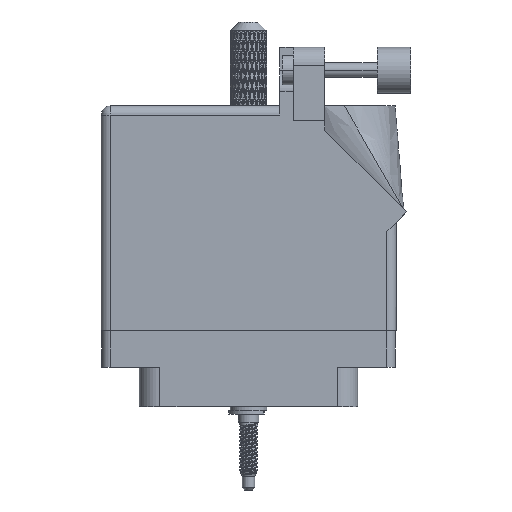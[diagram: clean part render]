
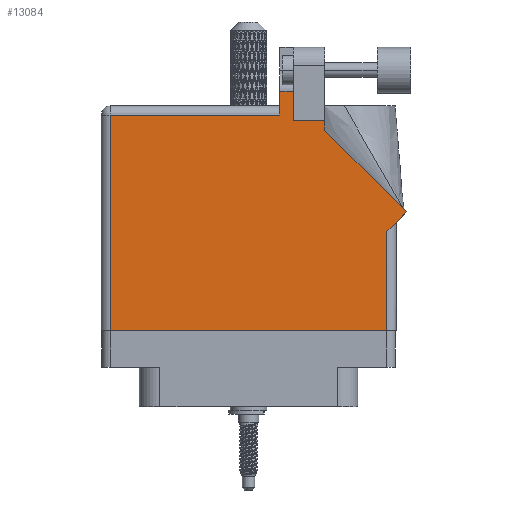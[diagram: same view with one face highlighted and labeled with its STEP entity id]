
A CAD part, front view. The second image highlights one B-rep face of the part: STEP entity #13084.
In plain terms, the highlighted face is planar.
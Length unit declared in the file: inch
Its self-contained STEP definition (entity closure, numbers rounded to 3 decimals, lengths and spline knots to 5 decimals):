
#128 = VERTEX_POINT ( 'NONE', #26891 ) ;
#2565 = EDGE_CURVE ( 'NONE', #128, #59512, #86111, .T. ) ;
#3086 = DIRECTION ( 'NONE',  ( 0.707, 0.707, 0. ) ) ;
#4726 = CARTESIAN_POINT ( 'NONE',  ( 0.519, 1.26442, 0.455 ) ) ;
#7536 = DIRECTION ( 'NONE',  ( 0., 0., -1. ) ) ;
#7722 = ORIENTED_EDGE ( 'NONE', *, *, #2565, .T. ) ;
#7923 = LINE ( 'NONE', #4726, #43890 ) ;
#8222 = LINE ( 'NONE', #74037, #45433 ) ;
#8623 = VECTOR ( 'NONE', #84389, 39.37008 ) ;
#8943 = EDGE_CURVE ( 'NONE', #104145, #89883, #28456, .T. ) ;
#11627 = EDGE_LOOP ( 'NONE', ( #90896, #99315, #51943, #72478, #7722, #75152, #79350, #53015, #60613, #103608, #106268 ) ) ;
#13084 = ADVANCED_FACE ( 'NONE', ( #33211 ), #72711, .F. ) ;
#14234 = CARTESIAN_POINT ( 'NONE',  ( 0.519, 1.33, 0.455 ) ) ;
#14616 = EDGE_CURVE ( 'NONE', #39354, #104145, #7923, .T. ) ;
#15587 = VECTOR ( 'NONE', #35825, 39.37008 ) ;
#15795 = DIRECTION ( 'NONE',  ( -1., 0., 0. ) ) ;
#16015 = EDGE_CURVE ( 'NONE', #94150, #39354, #99330, .T. ) ;
#16647 = EDGE_CURVE ( 'NONE', #42135, #82045, #8222, .T. ) ;
#16929 = CARTESIAN_POINT ( 'NONE',  ( 0.212, 1.368, 0.455 ) ) ;
#19706 = CARTESIAN_POINT ( 'NONE',  ( -0.943, -0.1, 0.455 ) ) ;
#22257 = VERTEX_POINT ( 'NONE', #84050 ) ;
#22921 = CARTESIAN_POINT ( 'NONE',  ( -1.005, 1.43, 0.455 ) ) ;
#24423 = EDGE_CURVE ( 'NONE', #89883, #22257, #54554, .T. ) ;
#24995 = DIRECTION ( 'NONE',  ( 0., 1., 0. ) ) ;
#25108 = EDGE_CURVE ( 'NONE', #73264, #42412, #90518, .T. ) ;
#26891 = CARTESIAN_POINT ( 'NONE',  ( -0.943, 1.368, 0.455 ) ) ;
#28456 = LINE ( 'NONE', #14234, #105423 ) ;
#32043 = CARTESIAN_POINT ( 'NONE',  ( 0.212, 1.43, 0.455 ) ) ;
#33211 = FACE_OUTER_BOUND ( 'NONE', #11627, .T. ) ;
#33916 = VECTOR ( 'NONE', #79499, 39.37008 ) ;
#35825 = DIRECTION ( 'NONE',  ( 0., -1., 0. ) ) ;
#36109 = EDGE_CURVE ( 'NONE', #82045, #94150, #38655, .T. ) ;
#37940 = VECTOR ( 'NONE', #40304, 39.37008 ) ;
#38655 = LINE ( 'NONE', #60293, #95187 ) ;
#39354 = VERTEX_POINT ( 'NONE', #59710 ) ;
#40304 = DIRECTION ( 'NONE',  ( 0., -1., 0. ) ) ;
#42135 = VERTEX_POINT ( 'NONE', #90522 ) ;
#42412 = VERTEX_POINT ( 'NONE', #16929 ) ;
#42532 = CARTESIAN_POINT ( 'NONE',  ( 1.07571, 0.70771, 0.455 ) ) ;
#43890 = VECTOR ( 'NONE', #70896, 39.37008 ) ;
#44619 = AXIS2_PLACEMENT_3D ( 'NONE', #22921, #7536, #15795 ) ;
#44699 = EDGE_CURVE ( 'NONE', #42412, #128, #81046, .T. ) ;
#45433 = VECTOR ( 'NONE', #24995, 39.37008 ) ;
#49109 = CARTESIAN_POINT ( 'NONE',  ( 0.306, 1.33, 0.455 ) ) ;
#49484 = VECTOR ( 'NONE', #56206, 39.37008 ) ;
#50236 = VECTOR ( 'NONE', #87895, 39.37008 ) ;
#50771 = CARTESIAN_POINT ( 'NONE',  ( 0.63677, 1.5315, 0.455 ) ) ;
#51943 = ORIENTED_EDGE ( 'NONE', *, *, #25108, .T. ) ;
#53015 = ORIENTED_EDGE ( 'NONE', *, *, #36109, .T. ) ;
#54554 = LINE ( 'NONE', #49109, #49484 ) ;
#56206 = DIRECTION ( 'NONE',  ( 0., 1., 0. ) ) ;
#59512 = VERTEX_POINT ( 'NONE', #92240 ) ;
#59710 = CARTESIAN_POINT ( 'NONE',  ( 0.519, 1.26442, 0.455 ) ) ;
#60293 = CARTESIAN_POINT ( 'NONE',  ( 1.005, 0.637, 0.455 ) ) ;
#60613 = ORIENTED_EDGE ( 'NONE', *, *, #16015, .T. ) ;
#65282 = DIRECTION ( 'NONE',  ( -1., 0., 0. ) ) ;
#65714 = EDGE_CURVE ( 'NONE', #59512, #42135, #95260, .T. ) ;
#70896 = DIRECTION ( 'NONE',  ( 0., 1., 0. ) ) ;
#72478 = ORIENTED_EDGE ( 'NONE', *, *, #44699, .T. ) ;
#72711 = PLANE ( 'NONE',  #44619 ) ;
#73264 = VERTEX_POINT ( 'NONE', #105266 ) ;
#74037 = CARTESIAN_POINT ( 'NONE',  ( 0.943, 0.637, 0.455 ) ) ;
#74223 = CARTESIAN_POINT ( 'NONE',  ( -1.005, 1.368, 0.455 ) ) ;
#75152 = ORIENTED_EDGE ( 'NONE', *, *, #65714, .T. ) ;
#79106 = EDGE_CURVE ( 'NONE', #22257, #73264, #80452, .T. ) ;
#79350 = ORIENTED_EDGE ( 'NONE', *, *, #16647, .T. ) ;
#79499 = DIRECTION ( 'NONE',  ( -0.707, 0.707, 0. ) ) ;
#80238 = CARTESIAN_POINT ( 'NONE',  ( 0.306, 1.33, 0.455 ) ) ;
#80452 = LINE ( 'NONE', #50771, #8623 ) ;
#81046 = LINE ( 'NONE', #74223, #90085 ) ;
#81148 = CARTESIAN_POINT ( 'NONE',  ( 0.943, 0.575, 0.455 ) ) ;
#82045 = VERTEX_POINT ( 'NONE', #81148 ) ;
#84050 = CARTESIAN_POINT ( 'NONE',  ( 0.306, 1.5315, 0.455 ) ) ;
#84389 = DIRECTION ( 'NONE',  ( -1., 0., 0. ) ) ;
#86111 = LINE ( 'NONE', #19706, #15587 ) ;
#86828 = CARTESIAN_POINT ( 'NONE',  ( -1.005, -0.1, 0.455 ) ) ;
#87895 = DIRECTION ( 'NONE',  ( 1., 0., 0. ) ) ;
#89883 = VERTEX_POINT ( 'NONE', #80238 ) ;
#90085 = VECTOR ( 'NONE', #65282, 39.37008 ) ;
#90518 = LINE ( 'NONE', #32043, #37940 ) ;
#90522 = CARTESIAN_POINT ( 'NONE',  ( 0.943, -0.1, 0.455 ) ) ;
#90896 = ORIENTED_EDGE ( 'NONE', *, *, #24423, .T. ) ;
#91318 = DIRECTION ( 'NONE',  ( -1., 0., 0. ) ) ;
#92240 = CARTESIAN_POINT ( 'NONE',  ( -0.943, -0.1, 0.455 ) ) ;
#94150 = VERTEX_POINT ( 'NONE', #42532 ) ;
#95187 = VECTOR ( 'NONE', #3086, 39.37008 ) ;
#95260 = LINE ( 'NONE', #86828, #50236 ) ;
#95415 = CARTESIAN_POINT ( 'NONE',  ( 1.07571, 0.70771, 0.455 ) ) ;
#99315 = ORIENTED_EDGE ( 'NONE', *, *, #79106, .T. ) ;
#99330 = LINE ( 'NONE', #95415, #33916 ) ;
#103608 = ORIENTED_EDGE ( 'NONE', *, *, #14616, .T. ) ;
#104145 = VERTEX_POINT ( 'NONE', #104916 ) ;
#104916 = CARTESIAN_POINT ( 'NONE',  ( 0.519, 1.33, 0.455 ) ) ;
#105266 = CARTESIAN_POINT ( 'NONE',  ( 0.212, 1.5315, 0.455 ) ) ;
#105423 = VECTOR ( 'NONE', #91318, 39.37008 ) ;
#106268 = ORIENTED_EDGE ( 'NONE', *, *, #8943, .T. ) ;
